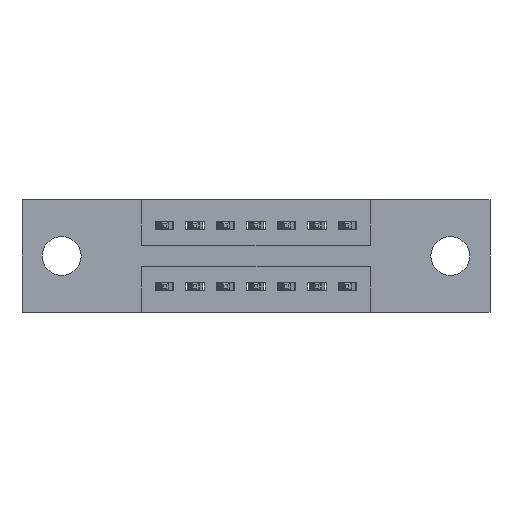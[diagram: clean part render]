
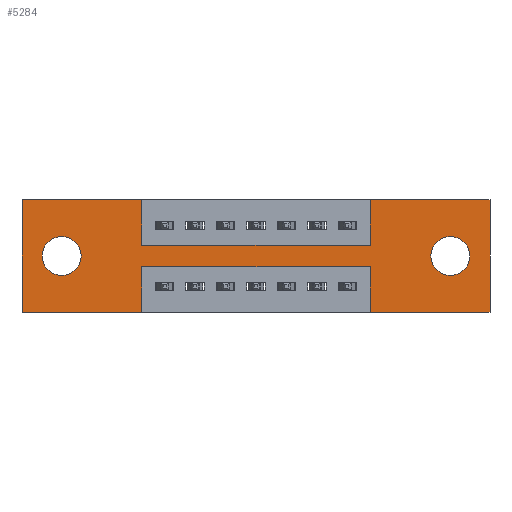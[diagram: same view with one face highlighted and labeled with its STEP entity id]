
A CAD part, front view. The second image highlights one B-rep face of the part: STEP entity #5284.
In plain terms, the highlighted planar face has unit normal (0, -1, 0).
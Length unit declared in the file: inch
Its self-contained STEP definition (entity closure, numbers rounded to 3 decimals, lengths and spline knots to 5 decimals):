
#12 = CARTESIAN_POINT ( 'NONE',  ( 0., 0., -0.37 ) ) ;
#196 = CARTESIAN_POINT ( 'NONE',  ( 0., 0., 0. ) ) ;
#226 = EDGE_CURVE ( 'NONE', #2552, #8596, #9452, .T. ) ;
#349 = EDGE_LOOP ( 'NONE', ( #3483, #6596, #4883, #5413, #2745, #3196, #7532, #6604, #5545, #4644, #5017, #7040 ) ) ;
#371 = DIRECTION ( 'NONE',  ( 0., 0., -1. ) ) ;
#375 = CARTESIAN_POINT ( 'NONE',  ( 0.13, 0., -0.185 ) ) ;
#501 = ORIENTED_EDGE ( 'NONE', *, *, #7955, .T. ) ;
#566 = DIRECTION ( 'NONE',  ( 0., 0., -1. ) ) ;
#568 = EDGE_CURVE ( 'NONE', #5858, #6606, #5731, .T. ) ;
#794 = VERTEX_POINT ( 'NONE', #5980 ) ;
#957 = AXIS2_PLACEMENT_3D ( 'NONE', #9281, #10133, #7683 ) ;
#989 = LINE ( 'NONE', #9933, #1366 ) ;
#1124 = EDGE_CURVE ( 'NONE', #8958, #1299, #4731, .T. ) ;
#1299 = VERTEX_POINT ( 'NONE', #5116 ) ;
#1366 = VECTOR ( 'NONE', #4512, 39.37008 ) ;
#1531 = DIRECTION ( 'NONE',  ( -1., 0., 0. ) ) ;
#1645 = EDGE_CURVE ( 'NONE', #8505, #5589, #2016, .T. ) ;
#1957 = CARTESIAN_POINT ( 'NONE',  ( 1.1425, 0., -0.37 ) ) ;
#1960 = ORIENTED_EDGE ( 'NONE', *, *, #4203, .T. ) ;
#1975 = CARTESIAN_POINT ( 'NONE',  ( 1.1425, 0., -0.15 ) ) ;
#2016 = LINE ( 'NONE', #4219, #10177 ) ;
#2074 = VERTEX_POINT ( 'NONE', #9392 ) ;
#2117 = AXIS2_PLACEMENT_3D ( 'NONE', #9035, #6608, #371 ) ;
#2163 = CARTESIAN_POINT ( 'NONE',  ( 0., 0., -0.37 ) ) ;
#2174 = CARTESIAN_POINT ( 'NONE',  ( 0., 0., 0. ) ) ;
#2307 = EDGE_CURVE ( 'NONE', #7753, #8505, #2749, .T. ) ;
#2540 = DIRECTION ( 'NONE',  ( 0., 0., -1. ) ) ;
#2552 = VERTEX_POINT ( 'NONE', #1975 ) ;
#2745 = ORIENTED_EDGE ( 'NONE', *, *, #1124, .F. ) ;
#2749 = LINE ( 'NONE', #196, #10040 ) ;
#2931 = FACE_OUTER_BOUND ( 'NONE', #349, .T. ) ;
#2975 = CARTESIAN_POINT ( 'NONE',  ( 0., 0., -0.37 ) ) ;
#3104 = EDGE_CURVE ( 'NONE', #6434, #3555, #6776, .T. ) ;
#3164 = LINE ( 'NONE', #9171, #6477 ) ;
#3196 = ORIENTED_EDGE ( 'NONE', *, *, #9409, .F. ) ;
#3263 = EDGE_CURVE ( 'NONE', #3555, #4963, #8242, .T. ) ;
#3277 = ORIENTED_EDGE ( 'NONE', *, *, #5933, .T. ) ;
#3453 = VECTOR ( 'NONE', #566, 39.37008 ) ;
#3455 = LINE ( 'NONE', #4862, #6626 ) ;
#3483 = ORIENTED_EDGE ( 'NONE', *, *, #9831, .F. ) ;
#3555 = VERTEX_POINT ( 'NONE', #8943 ) ;
#3814 = VECTOR ( 'NONE', #8404, 39.37008 ) ;
#3853 = CARTESIAN_POINT ( 'NONE',  ( 0., 0., -0.37 ) ) ;
#3980 = CARTESIAN_POINT ( 'NONE',  ( 0.13, 0., -0.249 ) ) ;
#4121 = DIRECTION ( 'NONE',  ( 1., 0., 0. ) ) ;
#4203 = EDGE_CURVE ( 'NONE', #6606, #5858, #4792, .T. ) ;
#4210 = VECTOR ( 'NONE', #6334, 39.37008 ) ;
#4219 = CARTESIAN_POINT ( 'NONE',  ( 0., 0., 0. ) ) ;
#4251 = EDGE_CURVE ( 'NONE', #5589, #6399, #3455, .T. ) ;
#4462 = DIRECTION ( 'NONE',  ( 1., 0., 0. ) ) ;
#4512 = DIRECTION ( 'NONE',  ( 1., 0., 0. ) ) ;
#4571 = EDGE_LOOP ( 'NONE', ( #6829, #1960 ) ) ;
#4644 = ORIENTED_EDGE ( 'NONE', *, *, #1645, .F. ) ;
#4731 = LINE ( 'NONE', #8132, #7433 ) ;
#4759 = VECTOR ( 'NONE', #6739, 39.37008 ) ;
#4792 = CIRCLE ( 'NONE', #957, 0.064 ) ;
#4826 = CARTESIAN_POINT ( 'NONE',  ( 0.3925, 0., 0. ) ) ;
#4862 = CARTESIAN_POINT ( 'NONE',  ( 0.3925, 0., 0. ) ) ;
#4883 = ORIENTED_EDGE ( 'NONE', *, *, #3104, .F. ) ;
#4922 = VECTOR ( 'NONE', #1531, 39.37008 ) ;
#4963 = VERTEX_POINT ( 'NONE', #7923 ) ;
#5017 = ORIENTED_EDGE ( 'NONE', *, *, #2307, .F. ) ;
#5057 = CARTESIAN_POINT ( 'NONE',  ( 1.1425, 0., 0. ) ) ;
#5116 = CARTESIAN_POINT ( 'NONE',  ( 1.535, 0., -0.37 ) ) ;
#5156 = CARTESIAN_POINT ( 'NONE',  ( 0.3925, 0., -0.37 ) ) ;
#5209 = DIRECTION ( 'NONE',  ( 0., 1., 0. ) ) ;
#5284 = ADVANCED_FACE ( 'NONE', ( #5378, #5885, #2931 ), #6788, .T. ) ;
#5316 = LINE ( 'NONE', #12, #4210 ) ;
#5378 = FACE_BOUND ( 'NONE', #10019, .T. ) ;
#5413 = ORIENTED_EDGE ( 'NONE', *, *, #8623, .F. ) ;
#5545 = ORIENTED_EDGE ( 'NONE', *, *, #4251, .F. ) ;
#5589 = VERTEX_POINT ( 'NONE', #4826 ) ;
#5647 = DIRECTION ( 'NONE',  ( 0., 0., -1. ) ) ;
#5731 = CIRCLE ( 'NONE', #9995, 0.064 ) ;
#5858 = VERTEX_POINT ( 'NONE', #7156 ) ;
#5885 = FACE_BOUND ( 'NONE', #4571, .T. ) ;
#5933 = EDGE_CURVE ( 'NONE', #794, #2074, #7099, .T. ) ;
#5980 = CARTESIAN_POINT ( 'NONE',  ( 1.405, 0., -0.121 ) ) ;
#6003 = EDGE_CURVE ( 'NONE', #6399, #2552, #3164, .T. ) ;
#6043 = CARTESIAN_POINT ( 'NONE',  ( 1.1425, 0., -0.37 ) ) ;
#6069 = CARTESIAN_POINT ( 'NONE',  ( 0.3925, 0., -0.37 ) ) ;
#6172 = CARTESIAN_POINT ( 'NONE',  ( 1.535, 0., 0. ) ) ;
#6334 = DIRECTION ( 'NONE',  ( -1., 0., 0. ) ) ;
#6399 = VERTEX_POINT ( 'NONE', #9827 ) ;
#6434 = VERTEX_POINT ( 'NONE', #1957 ) ;
#6477 = VECTOR ( 'NONE', #4462, 39.37008 ) ;
#6596 = ORIENTED_EDGE ( 'NONE', *, *, #3263, .F. ) ;
#6604 = ORIENTED_EDGE ( 'NONE', *, *, #6003, .F. ) ;
#6606 = VERTEX_POINT ( 'NONE', #3980 ) ;
#6608 = DIRECTION ( 'NONE',  ( 0., 1., 0. ) ) ;
#6626 = VECTOR ( 'NONE', #5647, 39.37008 ) ;
#6687 = DIRECTION ( 'NONE',  ( 0., 0., 1. ) ) ;
#6739 = DIRECTION ( 'NONE',  ( 0., 0., 1. ) ) ;
#6776 = LINE ( 'NONE', #6043, #3814 ) ;
#6788 = PLANE ( 'NONE',  #9028 ) ;
#6829 = ORIENTED_EDGE ( 'NONE', *, *, #568, .T. ) ;
#7040 = ORIENTED_EDGE ( 'NONE', *, *, #8842, .F. ) ;
#7099 = CIRCLE ( 'NONE', #2117, 0.064 ) ;
#7156 = CARTESIAN_POINT ( 'NONE',  ( 0.13, 0., -0.121 ) ) ;
#7433 = VECTOR ( 'NONE', #2540, 39.37008 ) ;
#7529 = DIRECTION ( 'NONE',  ( 0., 0., -1. ) ) ;
#7532 = ORIENTED_EDGE ( 'NONE', *, *, #226, .F. ) ;
#7683 = DIRECTION ( 'NONE',  ( 0., 0., 1. ) ) ;
#7753 = VERTEX_POINT ( 'NONE', #2163 ) ;
#7923 = CARTESIAN_POINT ( 'NONE',  ( 0.3925, 0., -0.22 ) ) ;
#7955 = EDGE_CURVE ( 'NONE', #2074, #794, #9551, .T. ) ;
#8059 = DIRECTION ( 'NONE',  ( 0., 0., 1. ) ) ;
#8122 = LINE ( 'NONE', #5156, #3453 ) ;
#8132 = CARTESIAN_POINT ( 'NONE',  ( 1.535, 0., 0. ) ) ;
#8137 = LINE ( 'NONE', #3853, #8879 ) ;
#8237 = DIRECTION ( 'NONE',  ( 0., 1., 0. ) ) ;
#8242 = LINE ( 'NONE', #9419, #4922 ) ;
#8356 = VERTEX_POINT ( 'NONE', #6069 ) ;
#8404 = DIRECTION ( 'NONE',  ( 0., 0., 1. ) ) ;
#8461 = DIRECTION ( 'NONE',  ( 0., -1., 0. ) ) ;
#8505 = VERTEX_POINT ( 'NONE', #2174 ) ;
#8596 = VERTEX_POINT ( 'NONE', #8637 ) ;
#8623 = EDGE_CURVE ( 'NONE', #1299, #6434, #5316, .T. ) ;
#8637 = CARTESIAN_POINT ( 'NONE',  ( 1.1425, 0., 0. ) ) ;
#8842 = EDGE_CURVE ( 'NONE', #8356, #7753, #8137, .T. ) ;
#8879 = VECTOR ( 'NONE', #9391, 39.37008 ) ;
#8943 = CARTESIAN_POINT ( 'NONE',  ( 1.1425, 0., -0.22 ) ) ;
#8958 = VERTEX_POINT ( 'NONE', #6172 ) ;
#9028 = AXIS2_PLACEMENT_3D ( 'NONE', #2975, #8461, #10087 ) ;
#9035 = CARTESIAN_POINT ( 'NONE',  ( 1.405, 0., -0.185 ) ) ;
#9171 = CARTESIAN_POINT ( 'NONE',  ( 0.3925, 0., -0.15 ) ) ;
#9180 = CARTESIAN_POINT ( 'NONE',  ( 1.405, 0., -0.185 ) ) ;
#9281 = CARTESIAN_POINT ( 'NONE',  ( 0.13, 0., -0.185 ) ) ;
#9389 = AXIS2_PLACEMENT_3D ( 'NONE', #9180, #5209, #7529 ) ;
#9391 = DIRECTION ( 'NONE',  ( -1., 0., 0. ) ) ;
#9392 = CARTESIAN_POINT ( 'NONE',  ( 1.405, 0., -0.249 ) ) ;
#9409 = EDGE_CURVE ( 'NONE', #8596, #8958, #989, .T. ) ;
#9419 = CARTESIAN_POINT ( 'NONE',  ( 0.3925, 0., -0.22 ) ) ;
#9452 = LINE ( 'NONE', #5057, #4759 ) ;
#9551 = CIRCLE ( 'NONE', #9389, 0.064 ) ;
#9827 = CARTESIAN_POINT ( 'NONE',  ( 0.3925, 0., -0.15 ) ) ;
#9831 = EDGE_CURVE ( 'NONE', #4963, #8356, #8122, .T. ) ;
#9933 = CARTESIAN_POINT ( 'NONE',  ( 0., 0., 0. ) ) ;
#9995 = AXIS2_PLACEMENT_3D ( 'NONE', #375, #8237, #6687 ) ;
#10019 = EDGE_LOOP ( 'NONE', ( #3277, #501 ) ) ;
#10040 = VECTOR ( 'NONE', #8059, 39.37008 ) ;
#10087 = DIRECTION ( 'NONE',  ( 0., 0., -1. ) ) ;
#10133 = DIRECTION ( 'NONE',  ( 0., 1., 0. ) ) ;
#10177 = VECTOR ( 'NONE', #4121, 39.37008 ) ;
